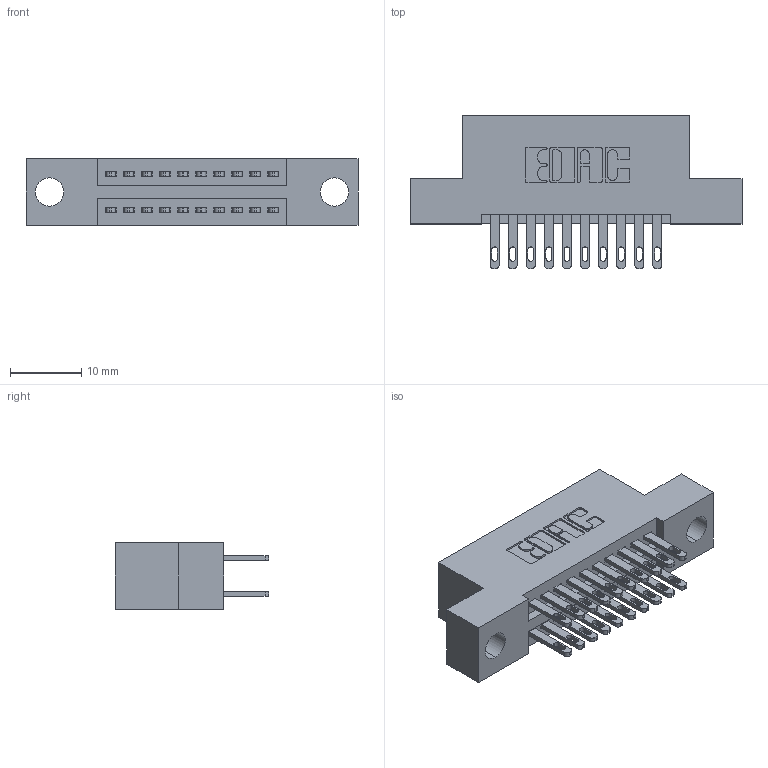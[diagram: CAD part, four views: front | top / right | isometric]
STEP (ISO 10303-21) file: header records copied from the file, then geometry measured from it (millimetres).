
FILE_DESCRIPTION (( 'STEP AP203' ), '1' );
FILE_NAME ('345-020-500-204.STEP', '2021-05-19T21:43:54', ( '' ), ( '' ), 'SwSTEP 2.0', 'SolidWorks 2020', '' );
FILE_SCHEMA (( 'CONFIG_CONTROL_DESIGN' ));
Length unit declared in the file: inch
Products named in the file (3): 345 Part_Flush Mounting Lugs - 0.156 Dia-TI; 345-292-001_345-293-100; 345-020-500-204
Assembly tree (21 placements, depth 2):
  345-020-500-204
    345 Part_Flush Mounting Lugs - 0.156 Dia-TI
    345-292-001_345-293-100  x20
Bounding box: 46.61 x 21.51 x 9.4 mm (x, y, z)
Volume: 4185.8 mm3; surface area: 5623.1 mm2
Topology: 21 solids, 21 shells, 1060 faces, 3197 edges, 2130 vertices
Faces by surface type: plane 634, cylinder 426
Entity records: 12503 total; most frequent: CARTESIAN_POINT 2130, ORIENTED_EDGE 2062, DIRECTION 1919, EDGE_CURVE 1031, LINE 855, VECTOR 855, VERTEX_POINT 686, AXIS2_PLACEMENT_3D 532
